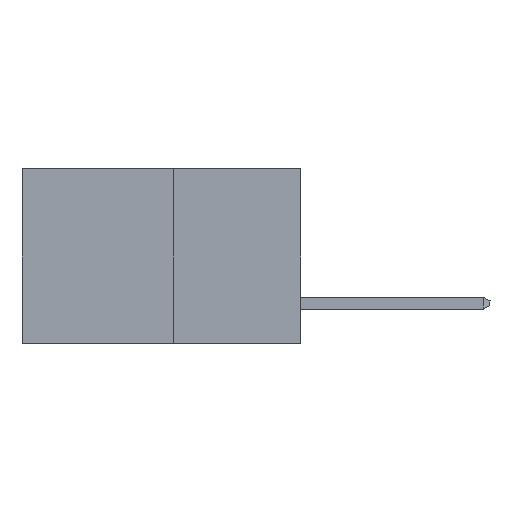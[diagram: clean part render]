
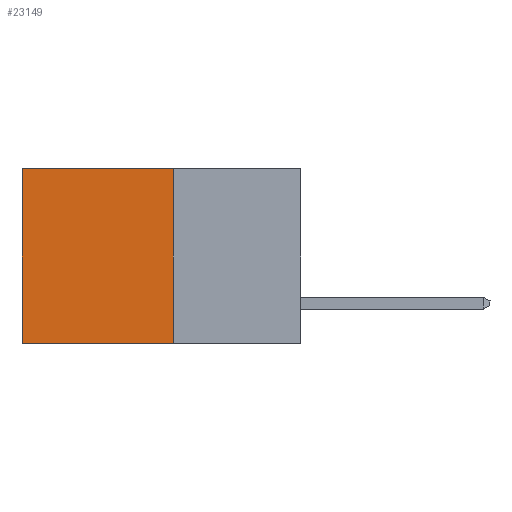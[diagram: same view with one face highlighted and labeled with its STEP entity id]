
A CAD part, left-side view. The second image highlights one B-rep face of the part: STEP entity #23149.
In plain terms, the highlighted planar face has unit normal (-1, 0, 0).
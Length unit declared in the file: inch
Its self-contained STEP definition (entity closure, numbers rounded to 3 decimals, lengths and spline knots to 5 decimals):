
#1149 = ORIENTED_EDGE ( 'NONE', *, *, #11809, .F. ) ;
#1273 = EDGE_CURVE ( 'NONE', #22284, #20400, #7697, .T. ) ;
#1288 = VERTEX_POINT ( 'NONE', #20054 ) ;
#1298 = LINE ( 'NONE', #2976, #10432 ) ;
#2833 = PLANE ( 'NONE',  #8672 ) ;
#2976 = CARTESIAN_POINT ( 'NONE',  ( 0.277, 0.27, -0.37 ) ) ;
#3192 = EDGE_CURVE ( 'NONE', #20400, #19446, #4201, .T. ) ;
#3981 = EDGE_CURVE ( 'NONE', #22284, #1288, #5690, .T. ) ;
#4201 = LINE ( 'NONE', #11342, #4789 ) ;
#4789 = VECTOR ( 'NONE', #11187, 39.37008 ) ;
#5119 = CARTESIAN_POINT ( 'NONE',  ( 0.277, 0.59, 0. ) ) ;
#5690 = LINE ( 'NONE', #20099, #20610 ) ;
#6571 = CARTESIAN_POINT ( 'NONE',  ( 0.277, 0.27, -0.37 ) ) ;
#6644 = DIRECTION ( 'NONE',  ( 0., 1., 0. ) ) ;
#7317 = CARTESIAN_POINT ( 'NONE',  ( 0.277, 0.27, 0. ) ) ;
#7697 = LINE ( 'NONE', #19226, #21476 ) ;
#8369 = DIRECTION ( 'NONE',  ( 1., 0., 0. ) ) ;
#8478 = FACE_OUTER_BOUND ( 'NONE', #18884, .T. ) ;
#8672 = AXIS2_PLACEMENT_3D ( 'NONE', #6571, #8369, #20974 ) ;
#9269 = DIRECTION ( 'NONE',  ( 0., 0., -1. ) ) ;
#10432 = VECTOR ( 'NONE', #6644, 39.37008 ) ;
#10838 = ORIENTED_EDGE ( 'NONE', *, *, #3192, .T. ) ;
#11107 = CARTESIAN_POINT ( 'NONE',  ( 0.277, 0.59, -0.37 ) ) ;
#11187 = DIRECTION ( 'NONE',  ( 0., 0., -1. ) ) ;
#11342 = CARTESIAN_POINT ( 'NONE',  ( 0.277, 0.59, -0.37 ) ) ;
#11809 = EDGE_CURVE ( 'NONE', #1288, #19446, #1298, .T. ) ;
#16571 = ORIENTED_EDGE ( 'NONE', *, *, #1273, .T. ) ;
#18884 = EDGE_LOOP ( 'NONE', ( #10838, #1149, #22559, #16571 ) ) ;
#19171 = DIRECTION ( 'NONE',  ( 0., 1., 0. ) ) ;
#19226 = CARTESIAN_POINT ( 'NONE',  ( 0.277, 0.27, 0. ) ) ;
#19446 = VERTEX_POINT ( 'NONE', #11107 ) ;
#20054 = CARTESIAN_POINT ( 'NONE',  ( 0.277, 0.27, -0.37 ) ) ;
#20099 = CARTESIAN_POINT ( 'NONE',  ( 0.277, 0.27, -0.37 ) ) ;
#20400 = VERTEX_POINT ( 'NONE', #5119 ) ;
#20610 = VECTOR ( 'NONE', #9269, 39.37008 ) ;
#20974 = DIRECTION ( 'NONE',  ( 0., 0., -1. ) ) ;
#21476 = VECTOR ( 'NONE', #19171, 39.37008 ) ;
#22284 = VERTEX_POINT ( 'NONE', #7317 ) ;
#22559 = ORIENTED_EDGE ( 'NONE', *, *, #3981, .F. ) ;
#23149 = ADVANCED_FACE ( 'NONE', ( #8478 ), #2833, .F. ) ;
